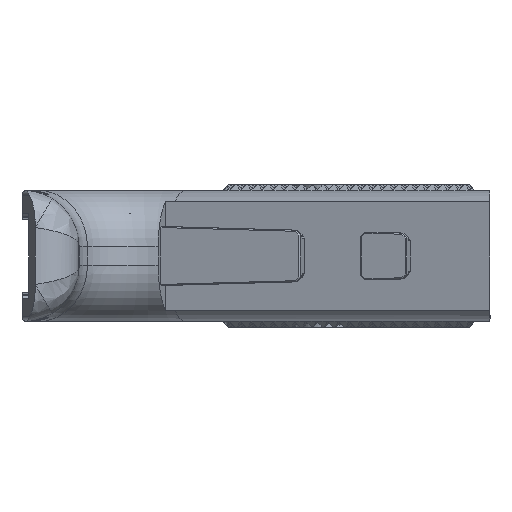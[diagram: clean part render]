
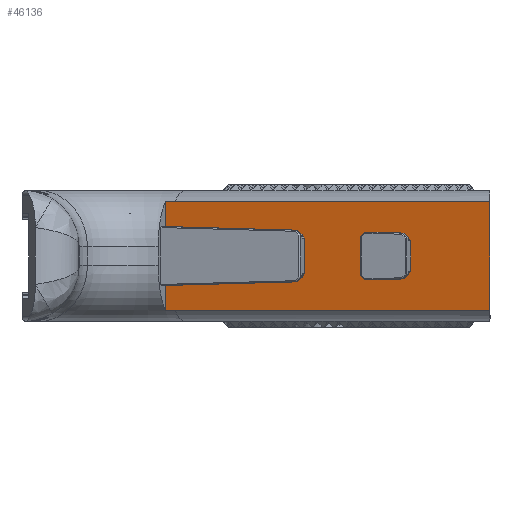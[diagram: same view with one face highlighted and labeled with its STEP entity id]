
A CAD part, left-side view. The second image highlights one B-rep face of the part: STEP entity #46136.
In plain terms, the highlighted planar face has unit normal (-0.951, 0.309, 0).
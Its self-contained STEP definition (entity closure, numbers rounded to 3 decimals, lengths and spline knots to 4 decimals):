
#54=FACE_BOUND('',#9105,.T.);
#731=B_SPLINE_CURVE_WITH_KNOTS('',3,(#88283,#88284,#88285,#88286,#88287,
#88288,#88289),.UNSPECIFIED.,.F.,.F.,(4,3,4),(0.,0.1181,0.2155),
 .UNSPECIFIED.);
#732=B_SPLINE_CURVE_WITH_KNOTS('',3,(#88297,#88298,#88299,#88300,#88301,
#88302,#88303),.UNSPECIFIED.,.F.,.F.,(4,3,4),(-0.2155,-0.1181,
0.),.UNSPECIFIED.);
#3339=PLANE('',#49166);
#6132=FACE_OUTER_BOUND('',#9104,.T.);
#9104=EDGE_LOOP('',(#41236,#41237,#41238,#41239,#41240,#41241,#41242,#41243,
#41244,#41245,#41246,#41247));
#9105=EDGE_LOOP('',(#41248,#41249,#41250,#41251,#41252,#41253,#41254,#41255,
#41256));
#14469=LINE('',#88172,#20011);
#14487=LINE('',#88210,#20029);
#14495=LINE('',#88227,#20037);
#14500=LINE('',#88236,#20042);
#14502=LINE('',#88239,#20044);
#14504=LINE('',#88244,#20046);
#14506=LINE('',#88248,#20048);
#14508=LINE('',#88251,#20050);
#14510=LINE('',#88255,#20052);
#14511=LINE('',#88257,#20053);
#14517=LINE('',#88270,#20059);
#14519=LINE('',#88274,#20061);
#14520=LINE('',#88277,#20062);
#14522=LINE('',#88281,#20064);
#14523=LINE('',#88291,#20065);
#14524=LINE('',#88293,#20066);
#14525=LINE('',#88295,#20067);
#14526=LINE('',#88305,#20068);
#14527=LINE('',#88306,#20069);
#20011=VECTOR('',#59728,0.3937);
#20029=VECTOR('',#59764,0.3937);
#20037=VECTOR('',#59778,0.3937);
#20042=VECTOR('',#59787,0.3937);
#20044=VECTOR('',#59791,0.3937);
#20046=VECTOR('',#59795,0.3937);
#20048=VECTOR('',#59799,0.3937);
#20050=VECTOR('',#59803,0.3937);
#20052=VECTOR('',#59807,0.3937);
#20053=VECTOR('',#59810,0.3937);
#20059=VECTOR('',#59826,0.3937);
#20061=VECTOR('',#59830,0.3937);
#20062=VECTOR('',#59833,0.3937);
#20064=VECTOR('',#59837,0.3937);
#20065=VECTOR('',#59838,0.3937);
#20066=VECTOR('',#59839,0.3937);
#20067=VECTOR('',#59840,0.3937);
#20068=VECTOR('',#59841,0.3937);
#20069=VECTOR('',#59842,0.3937);
#23558=VERTEX_POINT('',#88169);
#23559=VERTEX_POINT('',#88171);
#23569=VERTEX_POINT('',#88207);
#23570=VERTEX_POINT('',#88209);
#23575=VERTEX_POINT('',#88224);
#23576=VERTEX_POINT('',#88226);
#23578=VERTEX_POINT('',#88235);
#23579=VERTEX_POINT('',#88241);
#23580=VERTEX_POINT('',#88243);
#23581=VERTEX_POINT('',#88247);
#23582=VERTEX_POINT('',#88253);
#23584=VERTEX_POINT('',#88268);
#23585=VERTEX_POINT('',#88272);
#23586=VERTEX_POINT('',#88276);
#23587=VERTEX_POINT('',#88280);
#23588=VERTEX_POINT('',#88282);
#23589=VERTEX_POINT('',#88290);
#23590=VERTEX_POINT('',#88292);
#23591=VERTEX_POINT('',#88294);
#23592=VERTEX_POINT('',#88296);
#23593=VERTEX_POINT('',#88304);
#29547=EDGE_CURVE('',#23559,#23558,#14469,.T.);
#29565=EDGE_CURVE('',#23569,#23570,#14487,.T.);
#29573=EDGE_CURVE('',#23575,#23576,#14495,.F.);
#29578=EDGE_CURVE('',#23559,#23578,#14500,.F.);
#29580=EDGE_CURVE('',#23575,#23578,#14502,.T.);
#29582=EDGE_CURVE('',#23579,#23580,#14504,.F.);
#29584=EDGE_CURVE('',#23581,#23580,#14506,.T.);
#29586=EDGE_CURVE('',#23579,#23576,#14508,.T.);
#29588=EDGE_CURVE('',#23582,#23558,#14510,.F.);
#29589=EDGE_CURVE('',#23581,#23582,#14511,.F.);
#29595=EDGE_CURVE('',#23584,#23569,#14517,.F.);
#29597=EDGE_CURVE('',#23584,#23585,#14519,.T.);
#29598=EDGE_CURVE('',#23570,#23586,#14520,.F.);
#29600=EDGE_CURVE('',#23587,#23585,#14522,.T.);
#29601=EDGE_CURVE('',#23588,#23587,#731,.T.);
#29602=EDGE_CURVE('',#23589,#23588,#14523,.T.);
#29603=EDGE_CURVE('',#23590,#23589,#14524,.T.);
#29604=EDGE_CURVE('',#23591,#23590,#14525,.T.);
#29605=EDGE_CURVE('',#23592,#23591,#732,.T.);
#29606=EDGE_CURVE('',#23593,#23592,#14526,.T.);
#29607=EDGE_CURVE('',#23593,#23586,#14527,.T.);
#41236=ORIENTED_EDGE('',*,*,#29597,.T.);
#41237=ORIENTED_EDGE('',*,*,#29600,.F.);
#41238=ORIENTED_EDGE('',*,*,#29601,.F.);
#41239=ORIENTED_EDGE('',*,*,#29602,.F.);
#41240=ORIENTED_EDGE('',*,*,#29603,.F.);
#41241=ORIENTED_EDGE('',*,*,#29604,.F.);
#41242=ORIENTED_EDGE('',*,*,#29605,.F.);
#41243=ORIENTED_EDGE('',*,*,#29606,.F.);
#41244=ORIENTED_EDGE('',*,*,#29607,.T.);
#41245=ORIENTED_EDGE('',*,*,#29598,.F.);
#41246=ORIENTED_EDGE('',*,*,#29565,.F.);
#41247=ORIENTED_EDGE('',*,*,#29595,.F.);
#41248=ORIENTED_EDGE('',*,*,#29547,.T.);
#41249=ORIENTED_EDGE('',*,*,#29588,.F.);
#41250=ORIENTED_EDGE('',*,*,#29589,.F.);
#41251=ORIENTED_EDGE('',*,*,#29584,.T.);
#41252=ORIENTED_EDGE('',*,*,#29582,.F.);
#41253=ORIENTED_EDGE('',*,*,#29586,.T.);
#41254=ORIENTED_EDGE('',*,*,#29573,.F.);
#41255=ORIENTED_EDGE('',*,*,#29580,.T.);
#41256=ORIENTED_EDGE('',*,*,#29578,.F.);
#46136=ADVANCED_FACE('',(#6132,#54),#3339,.T.);
#49166=AXIS2_PLACEMENT_3D('',#88279,#59835,#59836);
#59728=DIRECTION('',(0.,0.,1.));
#59764=DIRECTION('',(0.,0.,1.));
#59778=DIRECTION('',(0.216,0.664,-0.716));
#59787=DIRECTION('',(0.221,0.681,0.698));
#59791=DIRECTION('',(0.309,0.951,-0.026));
#59795=DIRECTION('',(-0.216,-0.664,-0.716));
#59799=DIRECTION('',(-0.309,-0.951,-0.026));
#59803=DIRECTION('',(0.,0.,-1.));
#59807=DIRECTION('',(-0.12,-0.37,0.921));
#59810=DIRECTION('',(-0.221,-0.681,0.698));
#59826=DIRECTION('',(0.216,0.664,-0.716));
#59830=DIRECTION('',(0.309,0.951,-0.026));
#59833=DIRECTION('',(-0.216,-0.664,-0.716));
#59835=DIRECTION('center_axis',(-0.951,0.309,0.));
#59836=DIRECTION('ref_axis',(0.,0.,
1.));
#59837=DIRECTION('',(0.,0.,1.));
#59838=DIRECTION('',(0.309,0.951,0.));
#59839=DIRECTION('',(0.,0.,-1.));
#59840=DIRECTION('',(-0.309,-0.951,0.));
#59841=DIRECTION('',(0.,0.,1.));
#59842=DIRECTION('',(-0.309,-0.951,-0.026));
#88169=CARTESIAN_POINT('',(-2.8962,-0.8838,-0.6352));
#88171=CARTESIAN_POINT('',(-2.8962,-0.8838,-0.9101));
#88172=CARTESIAN_POINT('',(-2.8962,-0.8838,-0.7677));
#88207=CARTESIAN_POINT('',(-2.7262,-0.3607,-0.9245));
#88209=CARTESIAN_POINT('',(-2.7262,-0.3607,-0.6109));
#88210=CARTESIAN_POINT('',(-2.7262,-0.3607,-0.9154));
#88224=CARTESIAN_POINT('',(-3.0247,-1.2792,-0.909));
#88226=CARTESIAN_POINT('',(-3.0277,-1.2886,-0.8989));
#88227=CARTESIAN_POINT('',(-2.9908,-1.1749,-1.0217));
#88235=CARTESIAN_POINT('',(-2.8992,-0.8932,-0.9197));
#88236=CARTESIAN_POINT('',(-2.8709,-0.806,-0.8303));
#88239=CARTESIAN_POINT('',(-3.0469,-1.3476,-0.9072));
#88241=CARTESIAN_POINT('',(-3.0277,-1.2886,-0.6365));
#88243=CARTESIAN_POINT('',(-3.0247,-1.2792,-0.6264));
#88244=CARTESIAN_POINT('',(-2.9908,-1.1749,-0.5138));
#88247=CARTESIAN_POINT('',(-2.8992,-0.8932,-0.6158));
#88248=CARTESIAN_POINT('',(-3.0469,-1.3476,-0.6283));
#88251=CARTESIAN_POINT('',(-3.0277,-1.2886,-0.899));
#88253=CARTESIAN_POINT('',(-2.8984,-0.8905,-0.6185));
#88255=CARTESIAN_POINT('',(-2.885,-0.8493,-0.7213));
#88257=CARTESIAN_POINT('',(-2.8709,-0.806,-0.7051));
#88268=CARTESIAN_POINT('',(-2.7232,-0.3514,-0.9346));
#88270=CARTESIAN_POINT('',(-2.7647,-0.479,-0.7968));
#88272=CARTESIAN_POINT('',(-2.3324,0.8513,-0.9677));
#88274=CARTESIAN_POINT('',(-3.0469,-1.3476,-0.9072));
#88276=CARTESIAN_POINT('',(-2.7232,-0.3514,-0.6008));
#88277=CARTESIAN_POINT('',(-2.7647,-0.479,-0.7386));
#88279=CARTESIAN_POINT('Origin',(-2.8375,-0.7031,-0.7677));
#88280=CARTESIAN_POINT('',(-2.3324,0.8513,-1.2459));
#88281=CARTESIAN_POINT('',(-2.3324,0.8513,-1.0302));
#88282=CARTESIAN_POINT('',(-2.3592,0.7689,-1.2425));
#88283=CARTESIAN_POINT('Ctrl Pts',(-2.3592,0.7689,
-1.2425));
#88284=CARTESIAN_POINT('Ctrl Pts',(-2.3544,0.7836,
-1.2425));
#88285=CARTESIAN_POINT('Ctrl Pts',(-2.3495,0.7986,
-1.2428));
#88286=CARTESIAN_POINT('Ctrl Pts',(-2.3446,0.8138,
-1.2435));
#88287=CARTESIAN_POINT('Ctrl Pts',(-2.3405,0.8264,
-1.2441));
#88288=CARTESIAN_POINT('Ctrl Pts',(-2.3365,0.8388,
-1.2449));
#88289=CARTESIAN_POINT('Ctrl Pts',(-2.3324,0.8513,-1.2459));
#88290=CARTESIAN_POINT('',(-3.2516,-1.9775,-1.2425));
#88291=CARTESIAN_POINT('',(-2.1969,1.2684,-1.2425));
#88292=CARTESIAN_POINT('',(-3.2516,-1.9775,-0.2929));
#88293=CARTESIAN_POINT('',(-3.2516,-1.9775,-0.3839));
#88294=CARTESIAN_POINT('',(-2.3592,0.7689,-0.2929));
#88295=CARTESIAN_POINT('',(-2.6906,-0.2509,-0.2929));
#88296=CARTESIAN_POINT('',(-2.3324,0.8513,-0.2895));
#88297=CARTESIAN_POINT('Ctrl Pts',(-2.3324,0.8513,-0.2895));
#88298=CARTESIAN_POINT('Ctrl Pts',(-2.3365,0.8388,
-0.2905));
#88299=CARTESIAN_POINT('Ctrl Pts',(-2.3405,0.8264,
-0.2913));
#88300=CARTESIAN_POINT('Ctrl Pts',(-2.3446,0.8138,
-0.2919));
#88301=CARTESIAN_POINT('Ctrl Pts',(-2.3495,0.7986,
-0.2926));
#88302=CARTESIAN_POINT('Ctrl Pts',(-2.3544,0.7836,
-0.2929));
#88303=CARTESIAN_POINT('Ctrl Pts',(-2.3592,0.7689,
-0.2929));
#88304=CARTESIAN_POINT('',(-2.3324,0.8513,-0.5677));
#88305=CARTESIAN_POINT('',(-2.3324,0.8513,-0.7677));
#88306=CARTESIAN_POINT('',(-3.0469,-1.3476,-0.6283));
